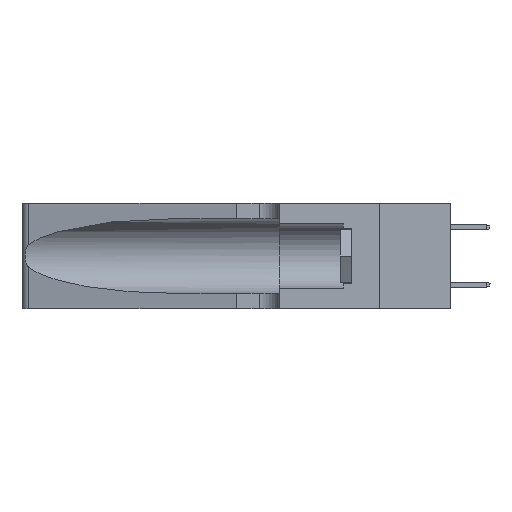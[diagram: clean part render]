
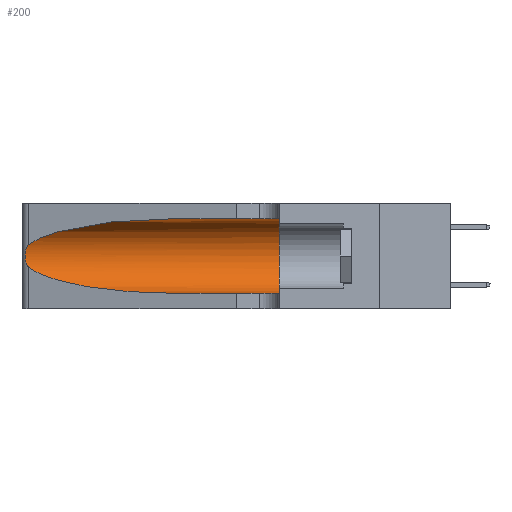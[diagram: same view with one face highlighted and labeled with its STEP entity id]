
A CAD part, left-side view. The second image highlights one B-rep face of the part: STEP entity #200.
In plain terms, the highlighted cylindrical face has radius 3.308 mm (diameter 6.617 mm), a partial arc.
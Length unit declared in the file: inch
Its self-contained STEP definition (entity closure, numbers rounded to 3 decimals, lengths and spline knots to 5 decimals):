
#200 = ADVANCED_FACE ( 'NONE', ( #3300 ), #12680, .F. ) ;
#426 = CARTESIAN_POINT ( 'NONE',  ( 0.25639, 1.23186, 0.15144 ) ) ;
#991 = DIRECTION ( 'NONE',  ( 0., 0., -1. ) ) ;
#1453 = CARTESIAN_POINT ( 'NONE',  ( 0.1305, 0.72297, 0.31525 ) ) ;
#3086 = CARTESIAN_POINT ( 'NONE',  ( 0.1305, 0.35, 0.05475 ) ) ;
#3300 = FACE_OUTER_BOUND ( 'NONE', #11535, .T. ) ;
#3770 = CARTESIAN_POINT ( 'NONE',  ( 0.1305, 0.72297, 0.05475 ) ) ;
#4060 = CARTESIAN_POINT ( 'NONE',  ( 0.25487, 1.22718, 0.14631 ) ) ;
#4259 = DIRECTION ( 'NONE',  ( 0., -1., 0. ) ) ;
#4610 = CARTESIAN_POINT ( 'NONE',  ( 0.25787, 1.23484, 0.2124 ) ) ;
#4624 = ORIENTED_EDGE ( 'NONE', *, *, #6798, .T. ) ;
#4655 = CARTESIAN_POINT ( 'NONE',  ( 0.1305, 0.72297, 0.31525 ) ) ;
#4729 = ORIENTED_EDGE ( 'NONE', *, *, #28317, .F. ) ;
#4754 = CARTESIAN_POINT ( 'NONE',  ( 0.26017, 1.23833, 0.17102 ) ) ;
#5045 = CARTESIAN_POINT ( 'NONE',  ( 0.25789, 1.23486, 0.15765 ) ) ;
#5073 = EDGE_CURVE ( 'NONE', #24031, #7208, #21278, .T. ) ;
#6117 = DIRECTION ( 'NONE',  ( 0., 1., 0. ) ) ;
#6444 = AXIS2_PLACEMENT_3D ( 'NONE', #18779, #25566, #991 ) ;
#6798 = EDGE_CURVE ( 'NONE', #7208, #18031, #14734, .T. ) ;
#7208 = VERTEX_POINT ( 'NONE', #24302 ) ;
#7384 = CARTESIAN_POINT ( 'NONE',  ( 0.25639, 1.23184, 0.21858 ) ) ;
#8201 = EDGE_CURVE ( 'NONE', #17039, #20091, #25146, .T. ) ;
#9144 = CARTESIAN_POINT ( 'NONE',  ( 0.26018, 1.23835, 0.19895 ) ) ;
#9574 = CARTESIAN_POINT ( 'NONE',  ( 0.25487, 1.22718, 0.14631 ) ) ;
#10062 = CARTESIAN_POINT ( 'NONE',  ( 0.2373, 1.15595, 0.08982 ) ) ;
#10220 = CARTESIAN_POINT ( 'NONE',  ( 0.2373, 1.15595, 0.28018 ) ) ;
#11316 = CARTESIAN_POINT ( 'NONE',  ( 0.1305, 0.35, 0.31525 ) ) ;
#11535 = EDGE_LOOP ( 'NONE', ( #24533, #25906, #26141, #4624, #4729, #16484 ) ) ;
#11718 = EDGE_CURVE ( 'NONE', #17039, #24552, #22346, .T. ) ;
#12113 = CIRCLE ( 'NONE', #27415, 0.13025 ) ;
#12680 = CYLINDRICAL_SURFACE ( 'NONE', #6444, 0.13025 ) ;
#12714 = DIRECTION ( 'NONE',  ( 0., -1., 0. ) ) ;
#12869 = DIRECTION ( 'NONE',  ( 0., 0., 1. ) ) ;
#13568 = CARTESIAN_POINT ( 'NONE',  ( 0.26075, 1.23896, 0.178 ) ) ;
#14281 = B_SPLINE_CURVE_WITH_KNOTS ( 'NONE', 3,
 ( #28534, #15890, #7384, #4610, #25151, #9144, #26896, #13568, #4754, #27181, #5045, #426, #27043, #9574 ),
 .UNSPECIFIED., .F., .F.,
 ( 4, 2, 2, 2, 2, 2, 4 ),
 ( 0., 0.00027, 0.00053, 0.00107, 0.0016, 0.00187, 0.00214 ),
 .UNSPECIFIED. ) ;
#14609 = CARTESIAN_POINT ( 'NONE',  ( 0.1305, 0.35, 0.185 ) ) ;
#14734 = LINE ( 'NONE', #23586, #16082 ) ;
#14740 = CARTESIAN_POINT ( 'NONE',  ( 0.25487, 1.22718, 0.22369 ) ) ;
#15890 = CARTESIAN_POINT ( 'NONE',  ( 0.25555, 1.22994, 0.2215 ) ) ;
#16082 = VECTOR ( 'NONE', #12714, 39.37008 ) ;
#16181 = VECTOR ( 'NONE', #4259, 39.37008 ) ;
#16482 = CARTESIAN_POINT ( 'NONE',  ( 0.18966, 0.96281, 0.31525 ) ) ;
#16484 = ORIENTED_EDGE ( 'NONE', *, *, #11718, .F. ) ;
#17039 = VERTEX_POINT ( 'NONE', #4655 ) ;
#18031 = VERTEX_POINT ( 'NONE', #3086 ) ;
#18779 = CARTESIAN_POINT ( 'NONE',  ( 0.1305, 1.61858, 0.185 ) ) ;
#20091 = VERTEX_POINT ( 'NONE', #25087 ) ;
#21278 =( BOUNDED_CURVE ( )  B_SPLINE_CURVE ( 3, ( #21723, #10062, #28088, #3770 ),
 .UNSPECIFIED., .F., .T. ) 
 B_SPLINE_CURVE_WITH_KNOTS ( ( 4, 4 ),
 ( 3.44316, 4.71239 ),
 .UNSPECIFIED. ) 
 CURVE ( )  GEOMETRIC_REPRESENTATION_ITEM ( )  RATIONAL_B_SPLINE_CURVE ( ( 1., 0.87, 0.87, 1. ) ) 
 REPRESENTATION_ITEM ( '' )  );
#21723 = CARTESIAN_POINT ( 'NONE',  ( 0.25487, 1.22718, 0.14631 ) ) ;
#22346 = LINE ( 'NONE', #24242, #16181 ) ;
#23586 = CARTESIAN_POINT ( 'NONE',  ( 0.1305, 1.61858, 0.05475 ) ) ;
#24031 = VERTEX_POINT ( 'NONE', #4060 ) ;
#24090 = EDGE_CURVE ( 'NONE', #20091, #24031, #14281, .T. ) ;
#24242 = CARTESIAN_POINT ( 'NONE',  ( 0.1305, 1.61858, 0.31525 ) ) ;
#24302 = CARTESIAN_POINT ( 'NONE',  ( 0.1305, 0.72297, 0.05475 ) ) ;
#24533 = ORIENTED_EDGE ( 'NONE', *, *, #8201, .T. ) ;
#24552 = VERTEX_POINT ( 'NONE', #11316 ) ;
#25087 = CARTESIAN_POINT ( 'NONE',  ( 0.25487, 1.22718, 0.22369 ) ) ;
#25146 =( BOUNDED_CURVE ( )  B_SPLINE_CURVE ( 3, ( #1453, #16482, #10220, #14740 ),
 .UNSPECIFIED., .F., .T. ) 
 B_SPLINE_CURVE_WITH_KNOTS ( ( 4, 4 ),
 ( 1.5708, 2.84003 ),
 .UNSPECIFIED. ) 
 CURVE ( )  GEOMETRIC_REPRESENTATION_ITEM ( )  RATIONAL_B_SPLINE_CURVE ( ( 1., 0.87, 0.87, 1. ) ) 
 REPRESENTATION_ITEM ( '' )  );
#25151 = CARTESIAN_POINT ( 'NONE',  ( 0.25854, 1.2359, 0.20912 ) ) ;
#25566 = DIRECTION ( 'NONE',  ( 0., -1., 0. ) ) ;
#25906 = ORIENTED_EDGE ( 'NONE', *, *, #24090, .T. ) ;
#26141 = ORIENTED_EDGE ( 'NONE', *, *, #5073, .T. ) ;
#26896 = CARTESIAN_POINT ( 'NONE',  ( 0.26075, 1.23896, 0.19203 ) ) ;
#27043 = CARTESIAN_POINT ( 'NONE',  ( 0.25555, 1.22993, 0.14849 ) ) ;
#27181 = CARTESIAN_POINT ( 'NONE',  ( 0.25856, 1.23593, 0.16098 ) ) ;
#27415 = AXIS2_PLACEMENT_3D ( 'NONE', #14609, #6117, #12869 ) ;
#28088 = CARTESIAN_POINT ( 'NONE',  ( 0.18966, 0.96281, 0.05475 ) ) ;
#28317 = EDGE_CURVE ( 'NONE', #24552, #18031, #12113, .T. ) ;
#28534 = CARTESIAN_POINT ( 'NONE',  ( 0.25487, 1.22718, 0.22369 ) ) ;
